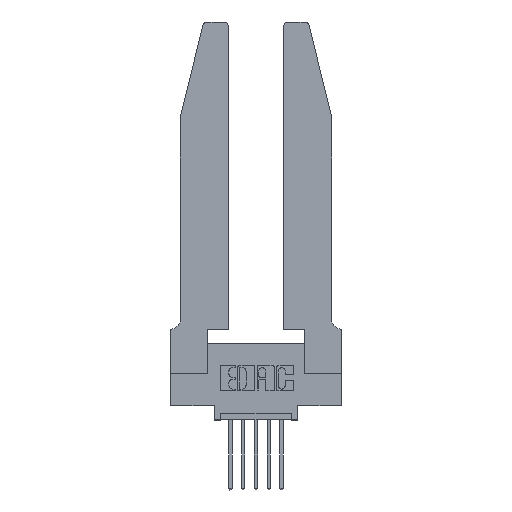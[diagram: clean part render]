
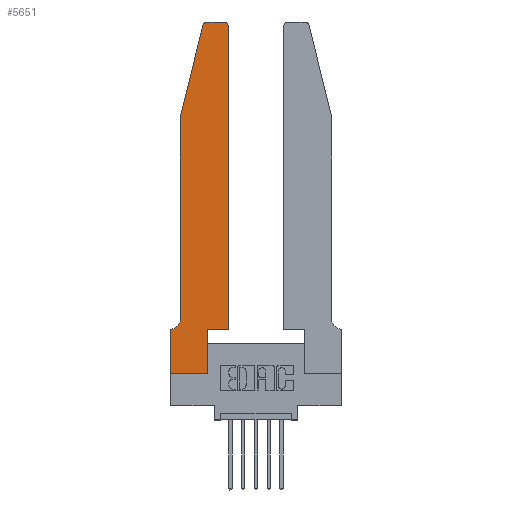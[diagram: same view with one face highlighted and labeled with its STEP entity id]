
A CAD part, top view. The second image highlights one B-rep face of the part: STEP entity #5651.
In plain terms, the highlighted planar face has unit normal (0, 0, 1).
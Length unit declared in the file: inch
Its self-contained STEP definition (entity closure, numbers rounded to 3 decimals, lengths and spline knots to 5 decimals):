
#103 = ORIENTED_EDGE ( 'NONE', *, *, #7435, .T. ) ;
#266 = AXIS2_PLACEMENT_3D ( 'NONE', #12296, #11843, #5661 ) ;
#627 = CARTESIAN_POINT ( 'NONE',  ( 0.2865, 0., 0.37 ) ) ;
#667 = VECTOR ( 'NONE', #5094, 39.37008 ) ;
#853 = ORIENTED_EDGE ( 'NONE', *, *, #7940, .T. ) ;
#937 = ORIENTED_EDGE ( 'NONE', *, *, #1801, .T. ) ;
#1024 = LINE ( 'NONE', #10493, #2506 ) ;
#1060 = AXIS2_PLACEMENT_3D ( 'NONE', #10601, #6412, #4476 ) ;
#1125 = EDGE_CURVE ( 'NONE', #2013, #7930, #11079, .T. ) ;
#1265 = CARTESIAN_POINT ( 'NONE',  ( 0.0055, 0.42, 0.37 ) ) ;
#1493 = EDGE_CURVE ( 'NONE', #4366, #13617, #6715, .T. ) ;
#1509 = VECTOR ( 'NONE', #11998, 39.37008 ) ;
#1567 = CARTESIAN_POINT ( 'NONE',  ( 0., 0.35, 0.37 ) ) ;
#1649 = CARTESIAN_POINT ( 'NONE',  ( 0.2865, 0.35, 0.37 ) ) ;
#1801 = EDGE_CURVE ( 'NONE', #11283, #10306, #4123, .T. ) ;
#1951 = CARTESIAN_POINT ( 'NONE',  ( 0.4205, 2.75, 0.37 ) ) ;
#2013 = VERTEX_POINT ( 'NONE', #2900 ) ;
#2080 = EDGE_CURVE ( 'NONE', #4533, #2013, #8705, .T. ) ;
#2179 = VECTOR ( 'NONE', #10290, 39.37008 ) ;
#2249 = EDGE_CURVE ( 'NONE', #10306, #6961, #5737, .T. ) ;
#2308 = VERTEX_POINT ( 'NONE', #627 ) ;
#2506 = VECTOR ( 'NONE', #4189, 39.37008 ) ;
#2613 = VERTEX_POINT ( 'NONE', #4542 ) ;
#2769 = ORIENTED_EDGE ( 'NONE', *, *, #1493, .T. ) ;
#2808 = CARTESIAN_POINT ( 'NONE',  ( 0.0755, 2., 0.37 ) ) ;
#2848 = DIRECTION ( 'NONE',  ( -0.239, -0.971, 0. ) ) ;
#2900 = CARTESIAN_POINT ( 'NONE',  ( 0.0055, 0.35, 0.37 ) ) ;
#2901 = ORIENTED_EDGE ( 'NONE', *, *, #7581, .T. ) ;
#3202 = EDGE_CURVE ( 'NONE', #9431, #5322, #10194, .T. ) ;
#3237 = DIRECTION ( 'NONE',  ( 0., -1., 0. ) ) ;
#3449 = ORIENTED_EDGE ( 'NONE', *, *, #3202, .T. ) ;
#3464 = VECTOR ( 'NONE', #4990, 39.37008 ) ;
#3473 = VECTOR ( 'NONE', #12690, 39.37008 ) ;
#3601 = LINE ( 'NONE', #5838, #5712 ) ;
#3626 = LINE ( 'NONE', #6171, #667 ) ;
#3881 = ORIENTED_EDGE ( 'NONE', *, *, #7146, .T. ) ;
#4123 = CIRCLE ( 'NONE', #1060, 0.03 ) ;
#4136 = CARTESIAN_POINT ( 'NONE',  ( 0., 0., 0.37 ) ) ;
#4189 = DIRECTION ( 'NONE',  ( -1., 0., 0. ) ) ;
#4366 = VERTEX_POINT ( 'NONE', #1649 ) ;
#4476 = DIRECTION ( 'NONE',  ( 1., 0., 0. ) ) ;
#4533 = VERTEX_POINT ( 'NONE', #7648 ) ;
#4542 = CARTESIAN_POINT ( 'NONE',  ( 0., 0., 0.37 ) ) ;
#4576 = DIRECTION ( 'NONE',  ( 0., 0., 1. ) ) ;
#4817 = CARTESIAN_POINT ( 'NONE',  ( 0.284, 2.75, 0.37 ) ) ;
#4839 = DIRECTION ( 'NONE',  ( 1., 0., 0. ) ) ;
#4990 = DIRECTION ( 'NONE',  ( 0., 1., 0. ) ) ;
#5016 = AXIS2_PLACEMENT_3D ( 'NONE', #1265, #8545, #11613 ) ;
#5094 = DIRECTION ( 'NONE',  ( 0., -1., 0. ) ) ;
#5103 = LINE ( 'NONE', #6554, #1509 ) ;
#5322 = VERTEX_POINT ( 'NONE', #1951 ) ;
#5623 = ORIENTED_EDGE ( 'NONE', *, *, #6567, .T. ) ;
#5651 = ADVANCED_FACE ( 'NONE', ( #8454 ), #13164, .T. ) ;
#5661 = DIRECTION ( 'NONE',  ( 1., 0., 0. ) ) ;
#5669 = ORIENTED_EDGE ( 'NONE', *, *, #1125, .T. ) ;
#5712 = VECTOR ( 'NONE', #4839, 39.37008 ) ;
#5737 = LINE ( 'NONE', #2808, #9872 ) ;
#5838 = CARTESIAN_POINT ( 'NONE',  ( 0., 0., 0.37 ) ) ;
#6171 = CARTESIAN_POINT ( 'NONE',  ( 0.0755, 2., 0.37 ) ) ;
#6412 = DIRECTION ( 'NONE',  ( 0., 0., 1. ) ) ;
#6542 = VECTOR ( 'NONE', #3237, 39.37008 ) ;
#6554 = CARTESIAN_POINT ( 'NONE',  ( 0.4505, 0.35, 0.37 ) ) ;
#6567 = EDGE_CURVE ( 'NONE', #5322, #11283, #1024, .T. ) ;
#6715 = LINE ( 'NONE', #10609, #3473 ) ;
#6783 = EDGE_LOOP ( 'NONE', ( #5623, #937, #11379, #853, #7064, #5669, #3881, #13024, #2901, #2769, #103, #3449 ) ) ;
#6961 = VERTEX_POINT ( 'NONE', #7028 ) ;
#7028 = CARTESIAN_POINT ( 'NONE',  ( 0.0755, 2., 0.37 ) ) ;
#7064 = ORIENTED_EDGE ( 'NONE', *, *, #2080, .T. ) ;
#7146 = EDGE_CURVE ( 'NONE', #7930, #2613, #13370, .T. ) ;
#7435 = EDGE_CURVE ( 'NONE', #13617, #9431, #5103, .T. ) ;
#7581 = EDGE_CURVE ( 'NONE', #2308, #4366, #8549, .T. ) ;
#7648 = CARTESIAN_POINT ( 'NONE',  ( 0.0755, 0.42, 0.37 ) ) ;
#7841 = CARTESIAN_POINT ( 'NONE',  ( 0.25487, 2.72718, 0.37 ) ) ;
#7930 = VERTEX_POINT ( 'NONE', #11552 ) ;
#7940 = EDGE_CURVE ( 'NONE', #6961, #4533, #3626, .T. ) ;
#8454 = FACE_OUTER_BOUND ( 'NONE', #6783, .T. ) ;
#8545 = DIRECTION ( 'NONE',  ( 0., 0., -1. ) ) ;
#8549 = LINE ( 'NONE', #10167, #3464 ) ;
#8705 = CIRCLE ( 'NONE', #5016, 0.07 ) ;
#8715 = CARTESIAN_POINT ( 'NONE',  ( 0.4505, 0.35, 0.37 ) ) ;
#8981 = EDGE_CURVE ( 'NONE', #2613, #2308, #3601, .T. ) ;
#9431 = VERTEX_POINT ( 'NONE', #13181 ) ;
#9872 = VECTOR ( 'NONE', #2848, 39.37008 ) ;
#9875 = DIRECTION ( 'NONE',  ( 1., 0., 0. ) ) ;
#10167 = CARTESIAN_POINT ( 'NONE',  ( 0.2865, 0.35, 0.37 ) ) ;
#10194 = CIRCLE ( 'NONE', #266, 0.03 ) ;
#10290 = DIRECTION ( 'NONE',  ( -1., 0., 0. ) ) ;
#10306 = VERTEX_POINT ( 'NONE', #7841 ) ;
#10493 = CARTESIAN_POINT ( 'NONE',  ( 0.2605, 2.75, 0.37 ) ) ;
#10601 = CARTESIAN_POINT ( 'NONE',  ( 0.284, 2.72, 0.37 ) ) ;
#10609 = CARTESIAN_POINT ( 'NONE',  ( 0.4505, 0.35, 0.37 ) ) ;
#11079 = LINE ( 'NONE', #11356, #2179 ) ;
#11283 = VERTEX_POINT ( 'NONE', #4817 ) ;
#11356 = CARTESIAN_POINT ( 'NONE',  ( 0.0755, 0.35, 0.37 ) ) ;
#11379 = ORIENTED_EDGE ( 'NONE', *, *, #2249, .T. ) ;
#11552 = CARTESIAN_POINT ( 'NONE',  ( 0., 0.35, 0.37 ) ) ;
#11613 = DIRECTION ( 'NONE',  ( -1., 0., 0. ) ) ;
#11843 = DIRECTION ( 'NONE',  ( 0., 0., 1. ) ) ;
#11998 = DIRECTION ( 'NONE',  ( 0., 1., 0. ) ) ;
#12276 = AXIS2_PLACEMENT_3D ( 'NONE', #1567, #4576, #9875 ) ;
#12296 = CARTESIAN_POINT ( 'NONE',  ( 0.4205, 2.72, 0.37 ) ) ;
#12690 = DIRECTION ( 'NONE',  ( 1., 0., 0. ) ) ;
#13024 = ORIENTED_EDGE ( 'NONE', *, *, #8981, .T. ) ;
#13164 = PLANE ( 'NONE',  #12276 ) ;
#13181 = CARTESIAN_POINT ( 'NONE',  ( 0.4505, 2.72, 0.37 ) ) ;
#13370 = LINE ( 'NONE', #4136, #6542 ) ;
#13617 = VERTEX_POINT ( 'NONE', #8715 ) ;
